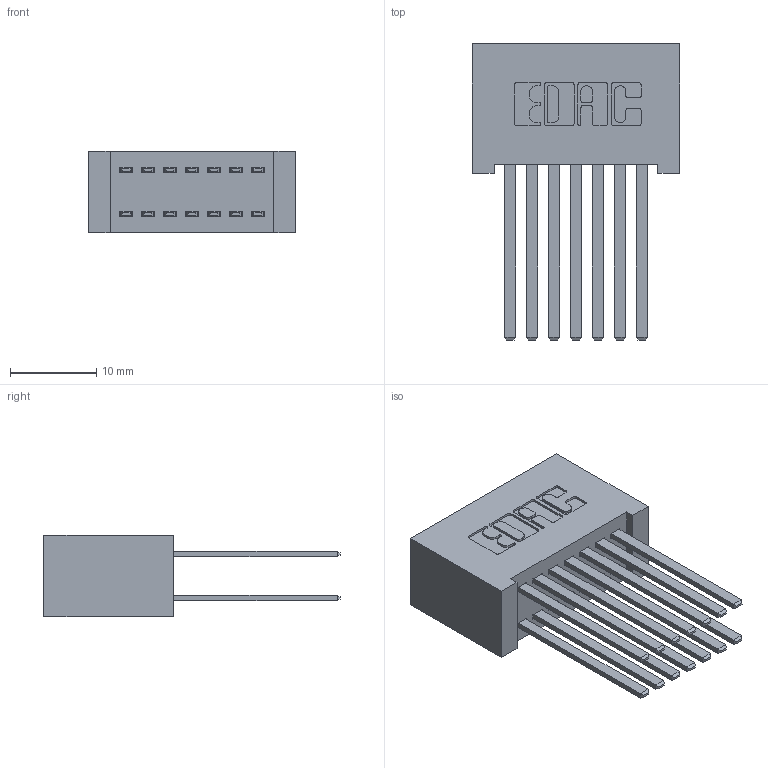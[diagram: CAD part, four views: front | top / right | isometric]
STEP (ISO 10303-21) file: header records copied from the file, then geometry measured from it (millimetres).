
FILE_DESCRIPTION (( 'STEP AP203' ), '1' );
FILE_NAME ('392-014-544-201.STEP', '2019-10-07T02:25:45', ( '' ), ( '' ), 'SwSTEP 2.0', 'SolidWorks 2016', '' );
FILE_SCHEMA (( 'CONFIG_CONTROL_DESIGN' ));
Length unit declared in the file: inch
Products named in the file (3): 342 Part_Lugless; 345-292-001_345-293-144; 392-014-544-201
Assembly tree (15 placements, depth 2):
  392-014-544-201
    342 Part_Lugless
    345-292-001_345-293-144  x14
Bounding box: 24.03 x 34.3 x 9.4 mm (x, y, z)
Volume: 2629 mm3; surface area: 4406.7 mm2
Topology: 15 solids, 15 shells, 746 faces, 2193 edges, 1442 vertices
Faces by surface type: plane 510, cylinder 236
Entity records: 8437 total; most frequent: CARTESIAN_POINT 1434, ORIENTED_EDGE 1370, DIRECTION 1277, EDGE_CURVE 685, VECTOR 569, LINE 569, VERTEX_POINT 454, AXIS2_PLACEMENT_3D 354
